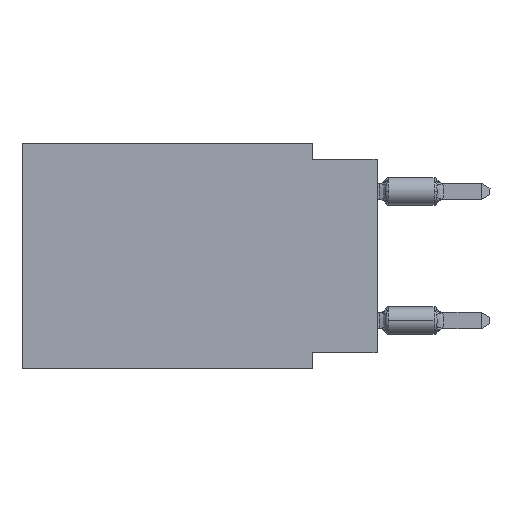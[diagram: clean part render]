
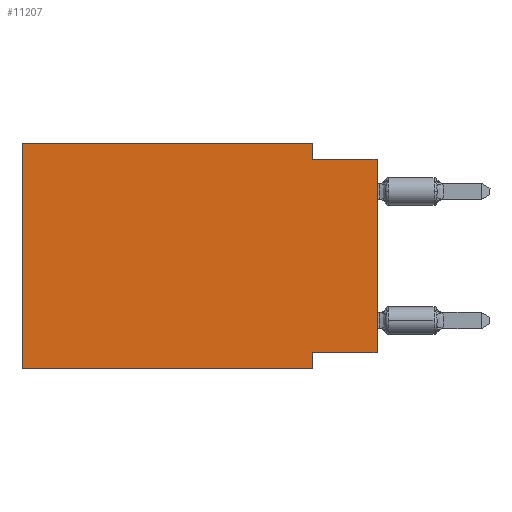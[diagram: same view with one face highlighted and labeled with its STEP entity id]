
A CAD part, left-side view. The second image highlights one B-rep face of the part: STEP entity #11207.
In plain terms, the highlighted planar face has unit normal (-1, 0, 0).
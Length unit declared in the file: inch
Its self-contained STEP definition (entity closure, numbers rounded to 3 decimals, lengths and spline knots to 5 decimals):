
#443 = VECTOR ( 'NONE', #1323, 39.37008 ) ;
#794 = EDGE_LOOP ( 'NONE', ( #1388, #9073, #4265, #1422, #12500, #1865, #7573, #6012 ) ) ;
#829 = EDGE_CURVE ( 'NONE', #6872, #4977, #13570, .T. ) ;
#1176 = VECTOR ( 'NONE', #14216, 39.37008 ) ;
#1269 = CARTESIAN_POINT ( 'NONE',  ( 0., 0.1, -0.35 ) ) ;
#1323 = DIRECTION ( 'NONE',  ( 0., 0., -1. ) ) ;
#1388 = ORIENTED_EDGE ( 'NONE', *, *, #11790, .T. ) ;
#1422 = ORIENTED_EDGE ( 'NONE', *, *, #2715, .F. ) ;
#1470 = CARTESIAN_POINT ( 'NONE',  ( 0., 0., -0.025 ) ) ;
#1865 = ORIENTED_EDGE ( 'NONE', *, *, #9514, .T. ) ;
#2165 = VECTOR ( 'NONE', #11998, 39.37008 ) ;
#2529 = DIRECTION ( 'NONE',  ( 0., -1., 0. ) ) ;
#2602 = AXIS2_PLACEMENT_3D ( 'NONE', #5411, #3107, #11233 ) ;
#2608 = CARTESIAN_POINT ( 'NONE',  ( 0., 0.55, 0. ) ) ;
#2715 = EDGE_CURVE ( 'NONE', #4977, #12395, #4267, .T. ) ;
#2836 = LINE ( 'NONE', #10644, #5566 ) ;
#3074 = EDGE_CURVE ( 'NONE', #4533, #3685, #12247, .T. ) ;
#3107 = DIRECTION ( 'NONE',  ( 1., 0., 0. ) ) ;
#3589 = VECTOR ( 'NONE', #5590, 39.37008 ) ;
#3685 = VERTEX_POINT ( 'NONE', #6679 ) ;
#4265 = ORIENTED_EDGE ( 'NONE', *, *, #7279, .F. ) ;
#4267 = LINE ( 'NONE', #2608, #1176 ) ;
#4415 = CARTESIAN_POINT ( 'NONE',  ( 0., 0., 0. ) ) ;
#4419 = CARTESIAN_POINT ( 'NONE',  ( 0., 0., -0.325 ) ) ;
#4461 = CARTESIAN_POINT ( 'NONE',  ( 0., 0., -0.025 ) ) ;
#4533 = VERTEX_POINT ( 'NONE', #14413 ) ;
#4880 = VERTEX_POINT ( 'NONE', #11574 ) ;
#4977 = VERTEX_POINT ( 'NONE', #10649 ) ;
#5047 = CARTESIAN_POINT ( 'NONE',  ( 0., 0.1, 0. ) ) ;
#5170 = VECTOR ( 'NONE', #9589, 39.37008 ) ;
#5411 = CARTESIAN_POINT ( 'NONE',  ( 0., 0.55, 0. ) ) ;
#5548 = CARTESIAN_POINT ( 'NONE',  ( 0., 0.1, -0.35 ) ) ;
#5566 = VECTOR ( 'NONE', #2529, 39.37008 ) ;
#5590 = DIRECTION ( 'NONE',  ( 0., 0., 1. ) ) ;
#5594 = DIRECTION ( 'NONE',  ( 0., 1., 0. ) ) ;
#6012 = ORIENTED_EDGE ( 'NONE', *, *, #3074, .F. ) ;
#6679 = CARTESIAN_POINT ( 'NONE',  ( 0., 0.1, -0.325 ) ) ;
#6872 = VERTEX_POINT ( 'NONE', #11190 ) ;
#7054 = CARTESIAN_POINT ( 'NONE',  ( 0., 0.55, 0. ) ) ;
#7279 = EDGE_CURVE ( 'NONE', #12395, #4880, #11067, .T. ) ;
#7433 = VECTOR ( 'NONE', #11670, 39.37008 ) ;
#7573 = ORIENTED_EDGE ( 'NONE', *, *, #14090, .F. ) ;
#7749 = PLANE ( 'NONE',  #2602 ) ;
#9073 = ORIENTED_EDGE ( 'NONE', *, *, #14193, .F. ) ;
#9514 = EDGE_CURVE ( 'NONE', #6872, #10425, #2836, .T. ) ;
#9589 = DIRECTION ( 'NONE',  ( 0., -1., 0. ) ) ;
#9702 = LINE ( 'NONE', #1269, #443 ) ;
#9778 = LINE ( 'NONE', #4415, #3589 ) ;
#10120 = CARTESIAN_POINT ( 'NONE',  ( 0., 0.1, 0. ) ) ;
#10425 = VERTEX_POINT ( 'NONE', #5548 ) ;
#10644 = CARTESIAN_POINT ( 'NONE',  ( 0., 0.55, -0.35 ) ) ;
#10649 = CARTESIAN_POINT ( 'NONE',  ( 0., 0.55, 0. ) ) ;
#11067 = LINE ( 'NONE', #5047, #2165 ) ;
#11190 = CARTESIAN_POINT ( 'NONE',  ( 0., 0.55, -0.35 ) ) ;
#11207 = ADVANCED_FACE ( 'NONE', ( #13484 ), #7749, .F. ) ;
#11233 = DIRECTION ( 'NONE',  ( 0., 0., -1. ) ) ;
#11574 = CARTESIAN_POINT ( 'NONE',  ( 0., 0.1, -0.025 ) ) ;
#11670 = DIRECTION ( 'NONE',  ( 0., 0., 1. ) ) ;
#11790 = EDGE_CURVE ( 'NONE', #4533, #14591, #9778, .T. ) ;
#11998 = DIRECTION ( 'NONE',  ( 0., 0., -1. ) ) ;
#12247 = LINE ( 'NONE', #4419, #14955 ) ;
#12395 = VERTEX_POINT ( 'NONE', #10120 ) ;
#12500 = ORIENTED_EDGE ( 'NONE', *, *, #829, .F. ) ;
#13484 = FACE_OUTER_BOUND ( 'NONE', #794, .T. ) ;
#13570 = LINE ( 'NONE', #7054, #7433 ) ;
#14090 = EDGE_CURVE ( 'NONE', #3685, #10425, #9702, .T. ) ;
#14193 = EDGE_CURVE ( 'NONE', #4880, #14591, #14405, .T. ) ;
#14216 = DIRECTION ( 'NONE',  ( 0., -1., 0. ) ) ;
#14405 = LINE ( 'NONE', #1470, #5170 ) ;
#14413 = CARTESIAN_POINT ( 'NONE',  ( 0., 0., -0.325 ) ) ;
#14591 = VERTEX_POINT ( 'NONE', #4461 ) ;
#14955 = VECTOR ( 'NONE', #5594, 39.37008 ) ;
